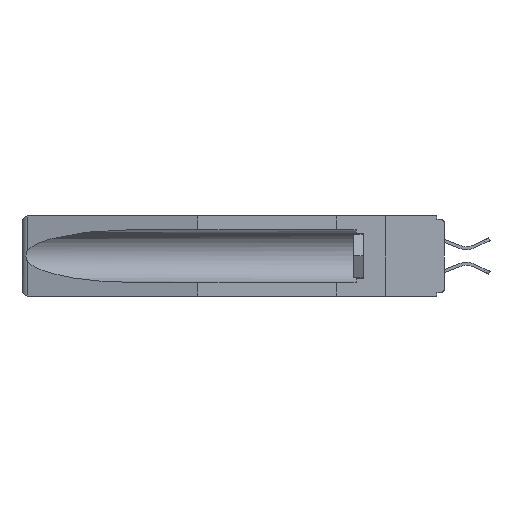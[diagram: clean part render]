
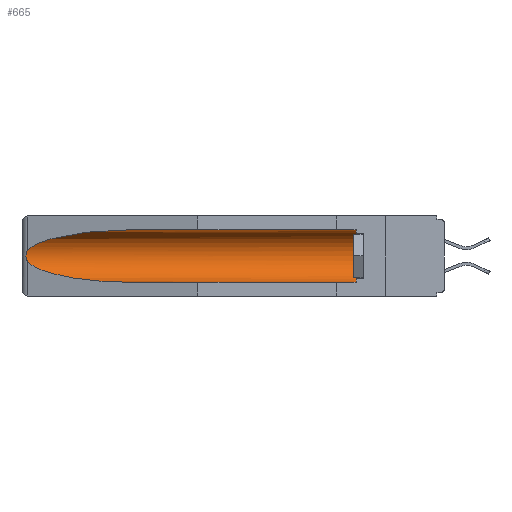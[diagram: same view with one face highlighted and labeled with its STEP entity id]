
A CAD part, left-side view. The second image highlights one B-rep face of the part: STEP entity #665.
In plain terms, the highlighted cylindrical face has radius 2.857 mm (diameter 5.715 mm), a partial arc.
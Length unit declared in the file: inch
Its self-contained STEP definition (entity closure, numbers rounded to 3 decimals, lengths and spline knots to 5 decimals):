
#119 = CARTESIAN_POINT ( 'NONE',  ( 0.26537, 1.52718, -0.19328 ) ) ;
#199 = VERTEX_POINT ( 'NONE', #10574 ) ;
#665 = ADVANCED_FACE ( 'NONE', ( #28302 ), #5501, .F. ) ;
#1436 = CARTESIAN_POINT ( 'NONE',  ( 0.26597, 1.52961, -0.15275 ) ) ;
#1491 = DIRECTION ( 'NONE',  ( 0., 1., 0. ) ) ;
#1549 = CARTESIAN_POINT ( 'NONE',  ( 0.2673, 1.5327, -0.16383 ) ) ;
#1563 = VECTOR ( 'NONE', #1491, 39.37008 ) ;
#2552 = AXIS2_PLACEMENT_3D ( 'NONE', #30757, #25794, #30445 ) ;
#4201 = LINE ( 'NONE', #6488, #1563 ) ;
#4995 = CARTESIAN_POINT ( 'NONE',  ( 0.25451, 1.48313, -0.24835 ) ) ;
#5205 = VERTEX_POINT ( 'NONE', #24452 ) ;
#5501 = CYLINDRICAL_SURFACE ( 'NONE', #28781, 0.1125 ) ;
#5717 = EDGE_CURVE ( 'NONE', #18688, #5205, #26556, .T. ) ;
#6196 = LINE ( 'NONE', #10731, #20412 ) ;
#6439 = B_SPLINE_CURVE_WITH_KNOTS ( 'NONE', 3,
 ( #25900, #1436, #16238, #1549, #13758, #23403, #28094, #28411, #26010, #10939 ),
 .UNSPECIFIED., .F., .F.,
 ( 4, 2, 2, 2, 4 ),
 ( 0., 0.00029, 0.00058, 0.00087, 0.00117 ),
 .UNSPECIFIED. ) ;
#6488 = CARTESIAN_POINT ( 'NONE',  ( 0.155, -0.30754, -0.059 ) ) ;
#6741 = ORIENTED_EDGE ( 'NONE', *, *, #28865, .T. ) ;
#7157 = EDGE_CURVE ( 'NONE', #23883, #18688, #4201, .T. ) ;
#9926 = CARTESIAN_POINT ( 'NONE',  ( 0.21114, 1.30732, -0.284 ) ) ;
#10574 = CARTESIAN_POINT ( 'NONE',  ( 0.155, 1.07973, -0.284 ) ) ;
#10731 = CARTESIAN_POINT ( 'NONE',  ( 0.155, -0.30754, -0.284 ) ) ;
#10939 = CARTESIAN_POINT ( 'NONE',  ( 0.26537, 1.52718, -0.19328 ) ) ;
#11289 = CARTESIAN_POINT ( 'NONE',  ( 0.155, 1.07973, -0.059 ) ) ;
#11816 = VERTEX_POINT ( 'NONE', #12308 ) ;
#12308 = CARTESIAN_POINT ( 'NONE',  ( 0.26537, 1.52718, -0.19328 ) ) ;
#12709 = EDGE_CURVE ( 'NONE', #5205, #11816, #6439, .T. ) ;
#13286 = ORIENTED_EDGE ( 'NONE', *, *, #18882, .T. ) ;
#13758 = CARTESIAN_POINT ( 'NONE',  ( 0.2675, 1.53308, -0.16763 ) ) ;
#16238 = CARTESIAN_POINT ( 'NONE',  ( 0.26654, 1.53092, -0.15636 ) ) ;
#16565 = CARTESIAN_POINT ( 'NONE',  ( 0.21114, 1.30732, -0.059 ) ) ;
#17656 = ORIENTED_EDGE ( 'NONE', *, *, #5717, .T. ) ;
#17728 = CARTESIAN_POINT ( 'NONE',  ( 0.155, 0.126, -0.059 ) ) ;
#18298 = DIRECTION ( 'NONE',  ( 0., 1., 0. ) ) ;
#18641 = CARTESIAN_POINT ( 'NONE',  ( 0.26537, 1.52718, -0.14972 ) ) ;
#18688 = VERTEX_POINT ( 'NONE', #20749 ) ;
#18847 = CARTESIAN_POINT ( 'NONE',  ( 0.25451, 1.48313, -0.09465 ) ) ;
#18882 = EDGE_CURVE ( 'NONE', #11816, #199, #30888, .T. ) ;
#19667 = DIRECTION ( 'NONE',  ( 0., 1., 0. ) ) ;
#19900 = ORIENTED_EDGE ( 'NONE', *, *, #30602, .F. ) ;
#20412 = VECTOR ( 'NONE', #18298, 39.37008 ) ;
#20462 = CIRCLE ( 'NONE', #2552, 0.1125 ) ;
#20749 = CARTESIAN_POINT ( 'NONE',  ( 0.155, 1.07973, -0.059 ) ) ;
#22060 = ORIENTED_EDGE ( 'NONE', *, *, #12709, .T. ) ;
#22722 = CARTESIAN_POINT ( 'NONE',  ( 0.155, 1.07973, -0.284 ) ) ;
#23403 = CARTESIAN_POINT ( 'NONE',  ( 0.2675, 1.53308, -0.17534 ) ) ;
#23883 = VERTEX_POINT ( 'NONE', #17728 ) ;
#23987 = CARTESIAN_POINT ( 'NONE',  ( 0.155, 0.126, -0.284 ) ) ;
#24452 = CARTESIAN_POINT ( 'NONE',  ( 0.26537, 1.52718, -0.14972 ) ) ;
#25794 = DIRECTION ( 'NONE',  ( 0., -1., 0. ) ) ;
#25900 = CARTESIAN_POINT ( 'NONE',  ( 0.26537, 1.52718, -0.14972 ) ) ;
#26010 = CARTESIAN_POINT ( 'NONE',  ( 0.26597, 1.5296, -0.19026 ) ) ;
#26080 = VERTEX_POINT ( 'NONE', #23987 ) ;
#26556 =( BOUNDED_CURVE ( )  B_SPLINE_CURVE ( 3, ( #11289, #16565, #18847, #18641 ),
 .UNSPECIFIED., .F., .F. ) 
 B_SPLINE_CURVE_WITH_KNOTS ( ( 4, 4 ),
 ( 4.71239, 6.08839 ),
 .UNSPECIFIED. ) 
 CURVE ( )  GEOMETRIC_REPRESENTATION_ITEM ( )  RATIONAL_B_SPLINE_CURVE ( ( 1., 0.848, 0.848, 1. ) ) 
 REPRESENTATION_ITEM ( '' )  );
#26935 = ORIENTED_EDGE ( 'NONE', *, *, #7157, .T. ) ;
#27159 = EDGE_LOOP ( 'NONE', ( #17656, #22060, #13286, #19900, #6741, #26935 ) ) ;
#28094 = CARTESIAN_POINT ( 'NONE',  ( 0.2673, 1.53269, -0.17917 ) ) ;
#28302 = FACE_OUTER_BOUND ( 'NONE', #27159, .T. ) ;
#28411 = CARTESIAN_POINT ( 'NONE',  ( 0.26655, 1.53094, -0.18657 ) ) ;
#28781 = AXIS2_PLACEMENT_3D ( 'NONE', #29083, #19667, #29181 ) ;
#28865 = EDGE_CURVE ( 'NONE', #26080, #23883, #20462, .T. ) ;
#29083 = CARTESIAN_POINT ( 'NONE',  ( 0.155, -0.30754, -0.1715 ) ) ;
#29181 = DIRECTION ( 'NONE',  ( 0., 0., 1. ) ) ;
#30445 = DIRECTION ( 'NONE',  ( 0., 0., 1. ) ) ;
#30602 = EDGE_CURVE ( 'NONE', #26080, #199, #6196, .T. ) ;
#30757 = CARTESIAN_POINT ( 'NONE',  ( 0.155, 0.126, -0.1715 ) ) ;
#30888 =( BOUNDED_CURVE ( )  B_SPLINE_CURVE ( 3, ( #119, #4995, #9926, #22722 ),
 .UNSPECIFIED., .F., .F. ) 
 B_SPLINE_CURVE_WITH_KNOTS ( ( 4, 4 ),
 ( 0.1948, 1.5708 ),
 .UNSPECIFIED. ) 
 CURVE ( )  GEOMETRIC_REPRESENTATION_ITEM ( )  RATIONAL_B_SPLINE_CURVE ( ( 1., 0.848, 0.848, 1. ) ) 
 REPRESENTATION_ITEM ( '' )  );
